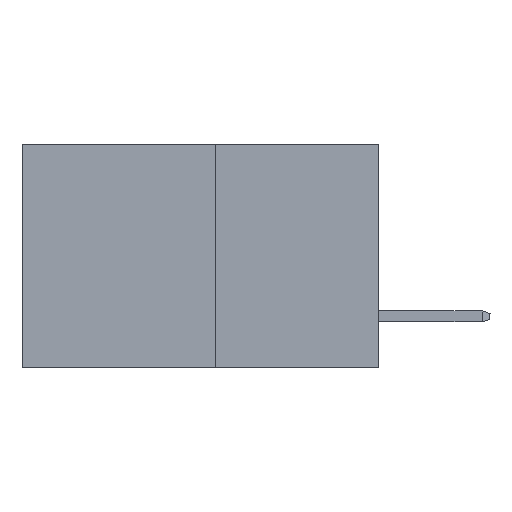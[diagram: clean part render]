
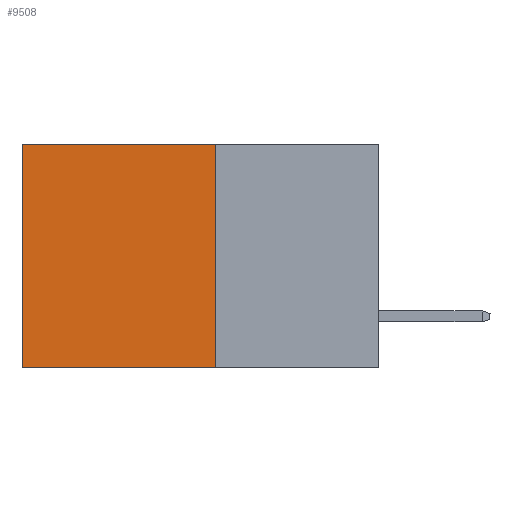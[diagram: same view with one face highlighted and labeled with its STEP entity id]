
A CAD part, left-side view. The second image highlights one B-rep face of the part: STEP entity #9508.
In plain terms, the highlighted planar face has unit normal (-1, 0, 0).
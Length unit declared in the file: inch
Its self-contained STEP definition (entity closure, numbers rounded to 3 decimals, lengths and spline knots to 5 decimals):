
#160 = EDGE_CURVE ( 'NONE', #5637, #14438, #5784, .T. ) ;
#469 = EDGE_CURVE ( 'NONE', #15873, #5637, #13016, .T. ) ;
#1528 = VECTOR ( 'NONE', #8728, 39.37008 ) ;
#2002 = VERTEX_POINT ( 'NONE', #11518 ) ;
#2477 = VECTOR ( 'NONE', #12347, 39.37008 ) ;
#2572 = ORIENTED_EDGE ( 'NONE', *, *, #15746, .T. ) ;
#3166 = CARTESIAN_POINT ( 'NONE',  ( 0.277, 0.27, -0.37 ) ) ;
#3185 = DIRECTION ( 'NONE',  ( 0., 0., -1. ) ) ;
#3716 = ORIENTED_EDGE ( 'NONE', *, *, #469, .F. ) ;
#4043 = DIRECTION ( 'NONE',  ( 0., 1., 0. ) ) ;
#5026 = CARTESIAN_POINT ( 'NONE',  ( 0.277, 0.27, -0.37 ) ) ;
#5228 = CARTESIAN_POINT ( 'NONE',  ( 0.277, 0.27, -0.37 ) ) ;
#5482 = FACE_OUTER_BOUND ( 'NONE', #14568, .T. ) ;
#5637 = VERTEX_POINT ( 'NONE', #5228 ) ;
#5784 = LINE ( 'NONE', #7696, #2477 ) ;
#6072 = LINE ( 'NONE', #12581, #15747 ) ;
#6263 = DIRECTION ( 'NONE',  ( 1., 0., 0. ) ) ;
#6938 = ORIENTED_EDGE ( 'NONE', *, *, #160, .F. ) ;
#7696 = CARTESIAN_POINT ( 'NONE',  ( 0.277, 0.27, -0.37 ) ) ;
#7739 = CARTESIAN_POINT ( 'NONE',  ( 0.277, 0.59, -0.37 ) ) ;
#8226 = LINE ( 'NONE', #14717, #1528 ) ;
#8728 = DIRECTION ( 'NONE',  ( 0., 0., -1. ) ) ;
#8875 = CARTESIAN_POINT ( 'NONE',  ( 0.277, 0.27, 0. ) ) ;
#9036 = AXIS2_PLACEMENT_3D ( 'NONE', #5026, #6263, #14760 ) ;
#9194 = EDGE_CURVE ( 'NONE', #15873, #2002, #6072, .T. ) ;
#9508 = ADVANCED_FACE ( 'NONE', ( #5482 ), #12348, .F. ) ;
#9816 = VECTOR ( 'NONE', #3185, 39.37008 ) ;
#11518 = CARTESIAN_POINT ( 'NONE',  ( 0.277, 0.59, 0. ) ) ;
#12347 = DIRECTION ( 'NONE',  ( 0., 1., 0. ) ) ;
#12348 = PLANE ( 'NONE',  #9036 ) ;
#12581 = CARTESIAN_POINT ( 'NONE',  ( 0.277, 0.27, 0. ) ) ;
#13016 = LINE ( 'NONE', #3166, #9816 ) ;
#13292 = ORIENTED_EDGE ( 'NONE', *, *, #9194, .T. ) ;
#14438 = VERTEX_POINT ( 'NONE', #7739 ) ;
#14568 = EDGE_LOOP ( 'NONE', ( #2572, #6938, #3716, #13292 ) ) ;
#14717 = CARTESIAN_POINT ( 'NONE',  ( 0.277, 0.59, -0.37 ) ) ;
#14760 = DIRECTION ( 'NONE',  ( 0., 0., -1. ) ) ;
#15746 = EDGE_CURVE ( 'NONE', #2002, #14438, #8226, .T. ) ;
#15747 = VECTOR ( 'NONE', #4043, 39.37008 ) ;
#15873 = VERTEX_POINT ( 'NONE', #8875 ) ;
